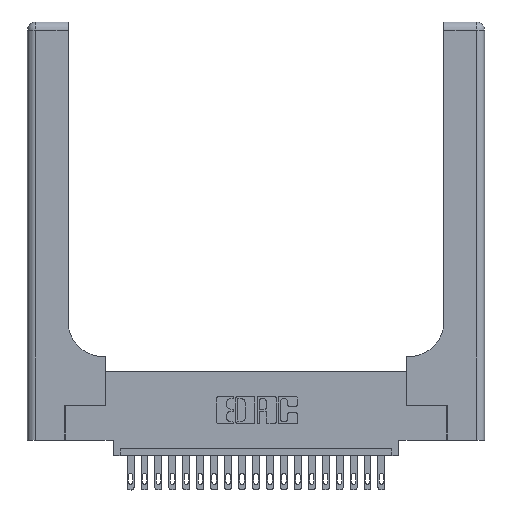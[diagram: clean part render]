
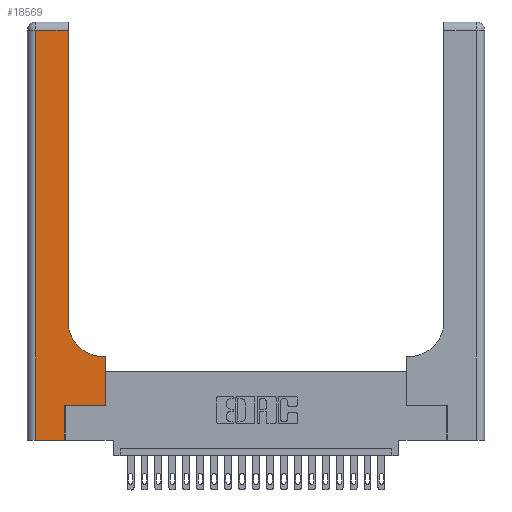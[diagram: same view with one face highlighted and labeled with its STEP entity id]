
A CAD part, top view. The second image highlights one B-rep face of the part: STEP entity #18569.
In plain terms, the highlighted planar face has unit normal (0, 0, 1).
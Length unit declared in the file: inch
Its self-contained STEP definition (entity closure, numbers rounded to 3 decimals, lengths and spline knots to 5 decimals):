
#217 = ORIENTED_EDGE ( 'NONE', *, *, #10550, .T. ) ;
#344 = VERTEX_POINT ( 'NONE', #3696 ) ;
#349 = CARTESIAN_POINT ( 'NONE',  ( 0.5585, 0.25, 0.37 ) ) ;
#921 = ORIENTED_EDGE ( 'NONE', *, *, #4435, .T. ) ;
#1506 = VERTEX_POINT ( 'NONE', #14929 ) ;
#1759 = VECTOR ( 'NONE', #14865, 39.37008 ) ;
#2404 = LINE ( 'NONE', #17135, #22086 ) ;
#2581 = CARTESIAN_POINT ( 'NONE',  ( 0.5585, 0.25, 0.37 ) ) ;
#3056 = VECTOR ( 'NONE', #7151, 39.37008 ) ;
#3483 = CARTESIAN_POINT ( 'NONE',  ( 0., 2.94, 0.37 ) ) ;
#3556 = CARTESIAN_POINT ( 'NONE',  ( 0.269, 0., 0.37 ) ) ;
#3568 = ORIENTED_EDGE ( 'NONE', *, *, #15043, .T. ) ;
#3696 = CARTESIAN_POINT ( 'NONE',  ( 0.2915, 0.85, 0.37 ) ) ;
#4023 = DIRECTION ( 'NONE',  ( 0., -1., 0. ) ) ;
#4286 = PLANE ( 'NONE',  #16520 ) ;
#4386 = EDGE_CURVE ( 'NONE', #4737, #14774, #21682, .T. ) ;
#4435 = EDGE_CURVE ( 'NONE', #14429, #1506, #18944, .T. ) ;
#4702 = EDGE_LOOP ( 'NONE', ( #7043, #9059, #3568, #217, #921, #5542, #16409, #10530, #19665 ) ) ;
#4704 = EDGE_CURVE ( 'NONE', #10004, #22652, #21414, .T. ) ;
#4737 = VERTEX_POINT ( 'NONE', #11369 ) ;
#5027 = DIRECTION ( 'NONE',  ( 0., 1., 0. ) ) ;
#5542 = ORIENTED_EDGE ( 'NONE', *, *, #9600, .T. ) ;
#5648 = VECTOR ( 'NONE', #18471, 39.37008 ) ;
#5669 = LINE ( 'NONE', #2581, #5648 ) ;
#5739 = DIRECTION ( 'NONE',  ( 1., 0., 0. ) ) ;
#6066 = DIRECTION ( 'NONE',  ( 0., 0., -1. ) ) ;
#6178 = CARTESIAN_POINT ( 'NONE',  ( 0.06, 0., 0.37 ) ) ;
#6835 = CARTESIAN_POINT ( 'NONE',  ( 0.06, 2.94, 0.37 ) ) ;
#7043 = ORIENTED_EDGE ( 'NONE', *, *, #12172, .T. ) ;
#7151 = DIRECTION ( 'NONE',  ( 1., 0., 0. ) ) ;
#7222 = LINE ( 'NONE', #7333, #18919 ) ;
#7333 = CARTESIAN_POINT ( 'NONE',  ( 0.269, 0.25, 0.37 ) ) ;
#7916 = FACE_OUTER_BOUND ( 'NONE', #4702, .T. ) ;
#8731 = CARTESIAN_POINT ( 'NONE',  ( 0., 0., 0.37 ) ) ;
#9059 = ORIENTED_EDGE ( 'NONE', *, *, #4386, .T. ) ;
#9274 = DIRECTION ( 'NONE',  ( 0., 0., -1. ) ) ;
#9600 = EDGE_CURVE ( 'NONE', #1506, #11061, #7222, .T. ) ;
#9676 = VECTOR ( 'NONE', #18964, 39.37008 ) ;
#10004 = VERTEX_POINT ( 'NONE', #19034 ) ;
#10530 = ORIENTED_EDGE ( 'NONE', *, *, #4704, .T. ) ;
#10550 = EDGE_CURVE ( 'NONE', #15758, #14429, #19662, .T. ) ;
#11061 = VERTEX_POINT ( 'NONE', #349 ) ;
#11369 = CARTESIAN_POINT ( 'NONE',  ( 0.2915, 2.94, 0.37 ) ) ;
#12172 = EDGE_CURVE ( 'NONE', #344, #4737, #2404, .T. ) ;
#12280 = DIRECTION ( 'NONE',  ( -1., 0., 0. ) ) ;
#12414 = CARTESIAN_POINT ( 'NONE',  ( 0.5415, 0.6, 0.37 ) ) ;
#12862 = DIRECTION ( 'NONE',  ( 1., 0., 0. ) ) ;
#13113 = CARTESIAN_POINT ( 'NONE',  ( 0.2915, 0.6, 0.37 ) ) ;
#14429 = VERTEX_POINT ( 'NONE', #21990 ) ;
#14774 = VERTEX_POINT ( 'NONE', #6835 ) ;
#14865 = DIRECTION ( 'NONE',  ( -1., 0., 0. ) ) ;
#14929 = CARTESIAN_POINT ( 'NONE',  ( 0.269, 0.25, 0.37 ) ) ;
#15043 = EDGE_CURVE ( 'NONE', #14774, #15758, #17092, .T. ) ;
#15758 = VERTEX_POINT ( 'NONE', #6178 ) ;
#16409 = ORIENTED_EDGE ( 'NONE', *, *, #21558, .T. ) ;
#16486 = CARTESIAN_POINT ( 'NONE',  ( 0., 3., 0.37 ) ) ;
#16520 = AXIS2_PLACEMENT_3D ( 'NONE', #16486, #6066, #18239 ) ;
#17092 = LINE ( 'NONE', #18140, #17620 ) ;
#17135 = CARTESIAN_POINT ( 'NONE',  ( 0.2915, 3., 0.37 ) ) ;
#17620 = VECTOR ( 'NONE', #4023, 39.37008 ) ;
#17677 = CIRCLE ( 'NONE', #19737, 0.25 ) ;
#18047 = CARTESIAN_POINT ( 'NONE',  ( 0.5415, 0.85, 0.37 ) ) ;
#18140 = CARTESIAN_POINT ( 'NONE',  ( 0.06, 3., 0.37 ) ) ;
#18239 = DIRECTION ( 'NONE',  ( -1., 0., 0. ) ) ;
#18409 = VECTOR ( 'NONE', #12280, 39.37008 ) ;
#18471 = DIRECTION ( 'NONE',  ( 0., 1., 0. ) ) ;
#18569 = ADVANCED_FACE ( 'NONE', ( #7916 ), #4286, .F. ) ;
#18919 = VECTOR ( 'NONE', #5739, 39.37008 ) ;
#18944 = LINE ( 'NONE', #3556, #9676 ) ;
#18964 = DIRECTION ( 'NONE',  ( 0., 1., 0. ) ) ;
#19034 = CARTESIAN_POINT ( 'NONE',  ( 0.5585, 0.6, 0.37 ) ) ;
#19662 = LINE ( 'NONE', #8731, #3056 ) ;
#19665 = ORIENTED_EDGE ( 'NONE', *, *, #20142, .T. ) ;
#19737 = AXIS2_PLACEMENT_3D ( 'NONE', #18047, #9274, #12862 ) ;
#20142 = EDGE_CURVE ( 'NONE', #22652, #344, #17677, .T. ) ;
#21414 = LINE ( 'NONE', #13113, #1759 ) ;
#21558 = EDGE_CURVE ( 'NONE', #11061, #10004, #5669, .T. ) ;
#21682 = LINE ( 'NONE', #3483, #18409 ) ;
#21990 = CARTESIAN_POINT ( 'NONE',  ( 0.269, 0., 0.37 ) ) ;
#22086 = VECTOR ( 'NONE', #5027, 39.37008 ) ;
#22652 = VERTEX_POINT ( 'NONE', #12414 ) ;
